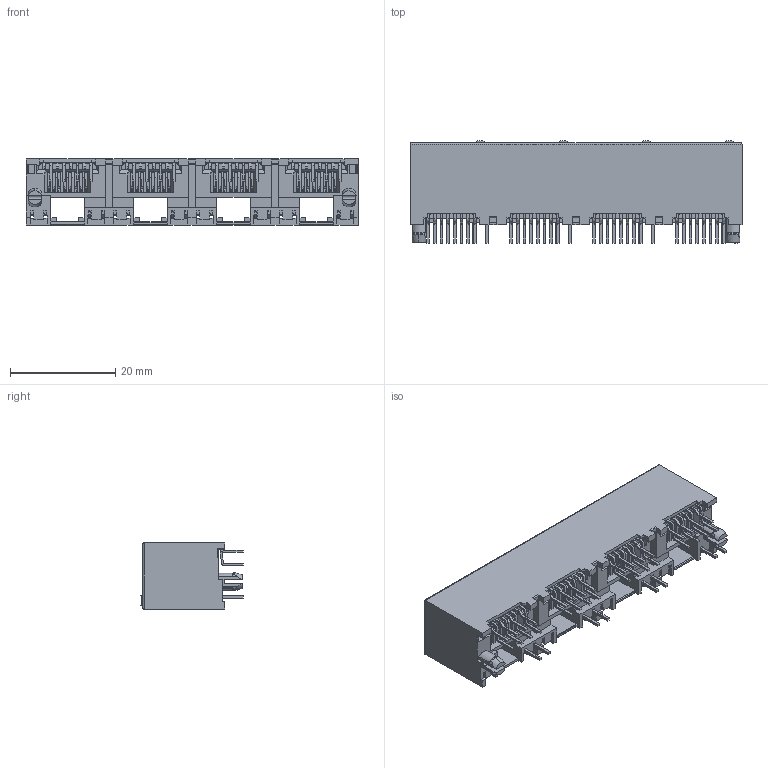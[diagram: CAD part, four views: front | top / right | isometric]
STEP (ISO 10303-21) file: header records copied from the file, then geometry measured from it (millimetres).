
FILE_DESCRIPTION (( 'STEP AP203' ), '1' );
FILE_NAME ('J2W048821N01031.STEP', '2020-10-05T19:55:03', ( '' ), ( '' ), 'SwSTEP 2.0', 'SolidWorks 2020', '' );
FILE_SCHEMA (( 'CONFIG_CONTROL_DESIGN' ));
Length unit declared in the file: millimetre
Products named in the file (6): 2W Insulator; 2W LED RH_1-Yellow; J2W048821N01031; 2W LED LH_0-Blank; 2W Contacts; 2W Contact Lock
Assembly tree (13 placements, depth 2):
  J2W048821N01031
    2W Insulator
    2W Contacts  x4
    2W Contact Lock  x4
    2W LED RH_1-Yellow  x4
  2W LED LH_0-Blank
Bounding box: 63 x 19.49 x 12.55 mm (x, y, z)
Volume: 5212.4 mm3; surface area: 12695.4 mm2
Topology: 41 solids, 41 shells, 3007 faces, 8830 edges, 5785 vertices
Faces by surface type: plane 2508, cylinder 441, bspline 47, cone 11
Entity records: 69198 total; most frequent: CARTESIAN_POINT 23723, ORIENTED_EDGE 11282, DIRECTION 6351, EDGE_CURVE 5641, VERTEX_POINT 3679, B_SPLINE_CURVE_WITH_KNOTS 3161, VECTOR 2297, LINE 2297
